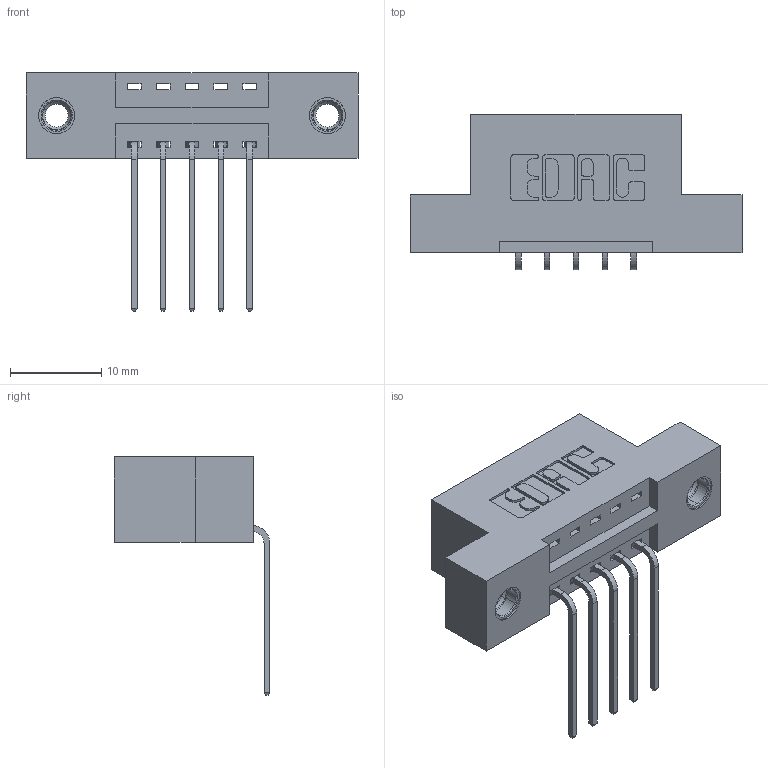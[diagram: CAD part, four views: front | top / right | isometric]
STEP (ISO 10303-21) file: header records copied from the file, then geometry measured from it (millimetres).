
FILE_DESCRIPTION (( 'STEP AP203' ), '1' );
FILE_NAME ('396-005-559-107.STEP', '2018-08-30T22:30:28', ( '' ), ( '' ), 'SwSTEP 2.0', 'SolidWorks 2016', '' );
FILE_SCHEMA (( 'CONFIG_CONTROL_DESIGN' ));
Length unit declared in the file: inch
Products named in the file (4): 346 Part_Flush Mounting Lugs - 0.156 Dia-TI; 345-292-001_558 559 Tail - 1; 345-250-001_345-250-005-103; 396-005-559-107
Assembly tree (8 placements, depth 2):
  396-005-559-107
    346 Part_Flush Mounting Lugs - 0.156 Dia-TI
    345-292-001_558 559 Tail - 1  x5
    345-250-001_345-250-005-103  x2
Bounding box: 36.45 x 17.08 x 26.16 mm (x, y, z)
Volume: 3237.2 mm3; surface area: 3780.8 mm2
Topology: 8 solids, 8 shells, 482 faces, 1375 edges, 902 vertices
Faces by surface type: plane 318, cylinder 148, cone 12, torus 4
Entity records: 9354 total; most frequent: CARTESIAN_POINT 1598, ORIENTED_EDGE 1530, DIRECTION 1481, EDGE_CURVE 765, LINE 593, VECTOR 593, VERTEX_POINT 504, AXIS2_PLACEMENT_3D 444
